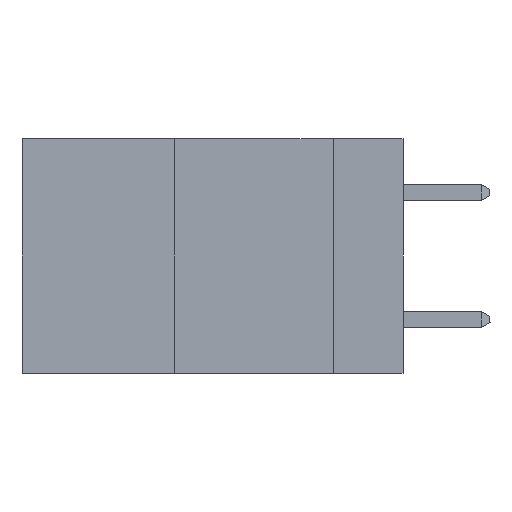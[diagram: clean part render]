
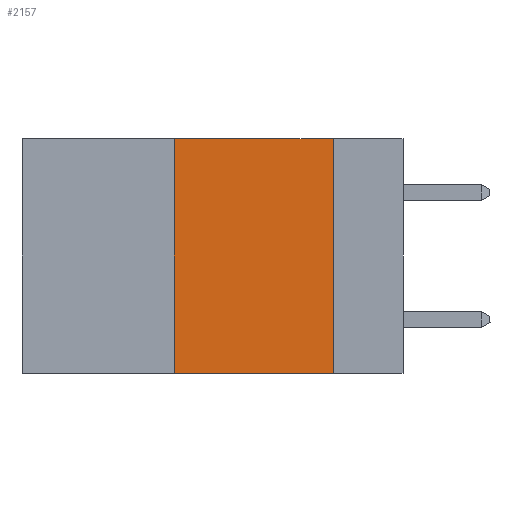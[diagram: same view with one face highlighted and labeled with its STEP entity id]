
A CAD part, left-side view. The second image highlights one B-rep face of the part: STEP entity #2157.
In plain terms, the highlighted planar face has unit normal (-1, 0, 0).
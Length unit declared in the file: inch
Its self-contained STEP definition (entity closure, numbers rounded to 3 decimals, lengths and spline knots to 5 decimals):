
#21 = VECTOR ( 'NONE', #7436, 39.37008 ) ;
#667 = EDGE_CURVE ( 'NONE', #13407, #16017, #3832, .T. ) ;
#1164 = ORIENTED_EDGE ( 'NONE', *, *, #12597, .F. ) ;
#2157 = ADVANCED_FACE ( 'NONE', ( #4410 ), #13828, .F. ) ;
#2412 = DIRECTION ( 'NONE',  ( 0., 0., 1. ) ) ;
#3035 = CARTESIAN_POINT ( 'NONE',  ( 0., 0.11, 0. ) ) ;
#3180 = EDGE_CURVE ( 'NONE', #7488, #5707, #9005, .T. ) ;
#3209 = VECTOR ( 'NONE', #2412, 39.37008 ) ;
#3256 = VECTOR ( 'NONE', #5649, 39.37008 ) ;
#3832 = LINE ( 'NONE', #4808, #21 ) ;
#4138 = ORIENTED_EDGE ( 'NONE', *, *, #13801, .F. ) ;
#4410 = FACE_OUTER_BOUND ( 'NONE', #4571, .T. ) ;
#4571 = EDGE_LOOP ( 'NONE', ( #1164, #8053, #4138, #8644 ) ) ;
#4808 = CARTESIAN_POINT ( 'NONE',  ( 0., 0.6, 0. ) ) ;
#5649 = DIRECTION ( 'NONE',  ( 0., 0., -1. ) ) ;
#5707 = VERTEX_POINT ( 'NONE', #16268 ) ;
#6183 = CARTESIAN_POINT ( 'NONE',  ( 0., 0.36, 0. ) ) ;
#6496 = DIRECTION ( 'NONE',  ( 0., -1., 0. ) ) ;
#6702 = LINE ( 'NONE', #3035, #3256 ) ;
#7436 = DIRECTION ( 'NONE',  ( 0., -1., 0. ) ) ;
#7488 = VERTEX_POINT ( 'NONE', #12283 ) ;
#8053 = ORIENTED_EDGE ( 'NONE', *, *, #667, .F. ) ;
#8644 = ORIENTED_EDGE ( 'NONE', *, *, #3180, .T. ) ;
#9005 = LINE ( 'NONE', #13001, #15524 ) ;
#11714 = LINE ( 'NONE', #6183, #3209 ) ;
#11876 = CARTESIAN_POINT ( 'NONE',  ( 0., 0.36, 0. ) ) ;
#12283 = CARTESIAN_POINT ( 'NONE',  ( 0., 0.36, -0.37 ) ) ;
#12310 = DIRECTION ( 'NONE',  ( 1., 0., 0. ) ) ;
#12597 = EDGE_CURVE ( 'NONE', #16017, #5707, #6702, .T. ) ;
#13001 = CARTESIAN_POINT ( 'NONE',  ( 0., 0.6, -0.37 ) ) ;
#13407 = VERTEX_POINT ( 'NONE', #11876 ) ;
#13780 = AXIS2_PLACEMENT_3D ( 'NONE', #15868, #12310, #16466 ) ;
#13801 = EDGE_CURVE ( 'NONE', #7488, #13407, #11714, .T. ) ;
#13828 = PLANE ( 'NONE',  #13780 ) ;
#13979 = CARTESIAN_POINT ( 'NONE',  ( 0., 0.11, 0. ) ) ;
#15524 = VECTOR ( 'NONE', #6496, 39.37008 ) ;
#15868 = CARTESIAN_POINT ( 'NONE',  ( 0., 0.6, 0. ) ) ;
#16017 = VERTEX_POINT ( 'NONE', #13979 ) ;
#16268 = CARTESIAN_POINT ( 'NONE',  ( 0., 0.11, -0.37 ) ) ;
#16466 = DIRECTION ( 'NONE',  ( 0., 0., -1. ) ) ;
